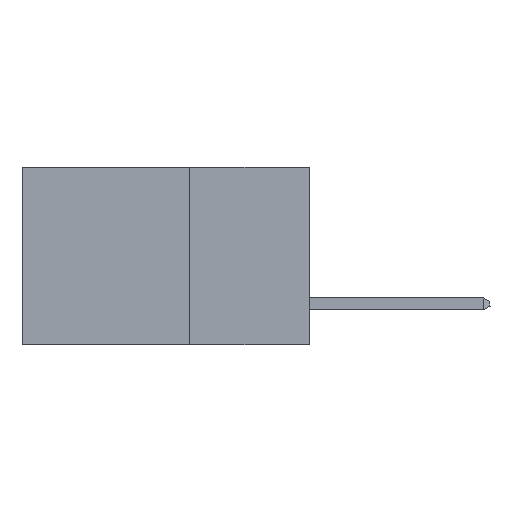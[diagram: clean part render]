
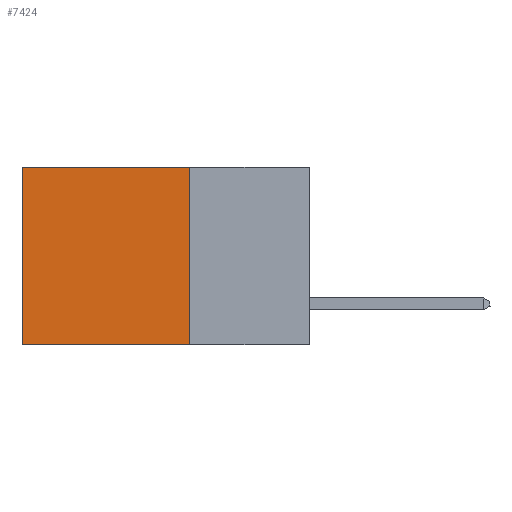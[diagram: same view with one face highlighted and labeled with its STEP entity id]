
A CAD part, left-side view. The second image highlights one B-rep face of the part: STEP entity #7424.
In plain terms, the highlighted planar face has unit normal (-1, 0, 0).
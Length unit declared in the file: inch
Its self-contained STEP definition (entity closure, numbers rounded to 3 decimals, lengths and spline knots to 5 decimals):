
#335 = VECTOR ( 'NONE', #534, 39.37008 ) ;
#534 = DIRECTION ( 'NONE',  ( 0., 1., 0. ) ) ;
#609 = EDGE_LOOP ( 'NONE', ( #16001, #13893, #10676, #13839 ) ) ;
#1072 = VERTEX_POINT ( 'NONE', #5575 ) ;
#1077 = CARTESIAN_POINT ( 'NONE',  ( 0.2875, 0.25, -0.37 ) ) ;
#1752 = CARTESIAN_POINT ( 'NONE',  ( 0.2875, 0.6, 0. ) ) ;
#1989 = DIRECTION ( 'NONE',  ( 0., 0., -1. ) ) ;
#3651 = LINE ( 'NONE', #5475, #335 ) ;
#4104 = VECTOR ( 'NONE', #14776, 39.37008 ) ;
#4322 = PLANE ( 'NONE',  #11568 ) ;
#4913 = CARTESIAN_POINT ( 'NONE',  ( 0.2875, 0.6, 0. ) ) ;
#5405 = DIRECTION ( 'NONE',  ( 1., 0., 0. ) ) ;
#5475 = CARTESIAN_POINT ( 'NONE',  ( 0.2875, 0.25, 0. ) ) ;
#5575 = CARTESIAN_POINT ( 'NONE',  ( 0.2875, 0.25, 0. ) ) ;
#6062 = DIRECTION ( 'NONE',  ( 0., 0., -1. ) ) ;
#6612 = EDGE_CURVE ( 'NONE', #1072, #11044, #3651, .T. ) ;
#7424 = ADVANCED_FACE ( 'NONE', ( #15481 ), #4322, .F. ) ;
#8285 = EDGE_CURVE ( 'NONE', #11521, #16073, #14018, .T. ) ;
#9262 = CARTESIAN_POINT ( 'NONE',  ( 0.2875, 0.25, 0. ) ) ;
#9438 = EDGE_CURVE ( 'NONE', #1072, #11521, #12237, .T. ) ;
#10083 = LINE ( 'NONE', #4913, #10484 ) ;
#10362 = EDGE_CURVE ( 'NONE', #11044, #16073, #10083, .T. ) ;
#10431 = DIRECTION ( 'NONE',  ( 0., 0., -1. ) ) ;
#10484 = VECTOR ( 'NONE', #6062, 39.37008 ) ;
#10676 = ORIENTED_EDGE ( 'NONE', *, *, #9438, .F. ) ;
#11044 = VERTEX_POINT ( 'NONE', #1752 ) ;
#11210 = CARTESIAN_POINT ( 'NONE',  ( 0.2875, 0.6, -0.37 ) ) ;
#11521 = VERTEX_POINT ( 'NONE', #15209 ) ;
#11568 = AXIS2_PLACEMENT_3D ( 'NONE', #12883, #5405, #10431 ) ;
#12237 = LINE ( 'NONE', #9262, #13407 ) ;
#12883 = CARTESIAN_POINT ( 'NONE',  ( 0.2875, 0.25, 0. ) ) ;
#13407 = VECTOR ( 'NONE', #1989, 39.37008 ) ;
#13839 = ORIENTED_EDGE ( 'NONE', *, *, #6612, .T. ) ;
#13893 = ORIENTED_EDGE ( 'NONE', *, *, #8285, .F. ) ;
#14018 = LINE ( 'NONE', #1077, #4104 ) ;
#14776 = DIRECTION ( 'NONE',  ( 0., 1., 0. ) ) ;
#15209 = CARTESIAN_POINT ( 'NONE',  ( 0.2875, 0.25, -0.37 ) ) ;
#15481 = FACE_OUTER_BOUND ( 'NONE', #609, .T. ) ;
#16001 = ORIENTED_EDGE ( 'NONE', *, *, #10362, .T. ) ;
#16073 = VERTEX_POINT ( 'NONE', #11210 ) ;
